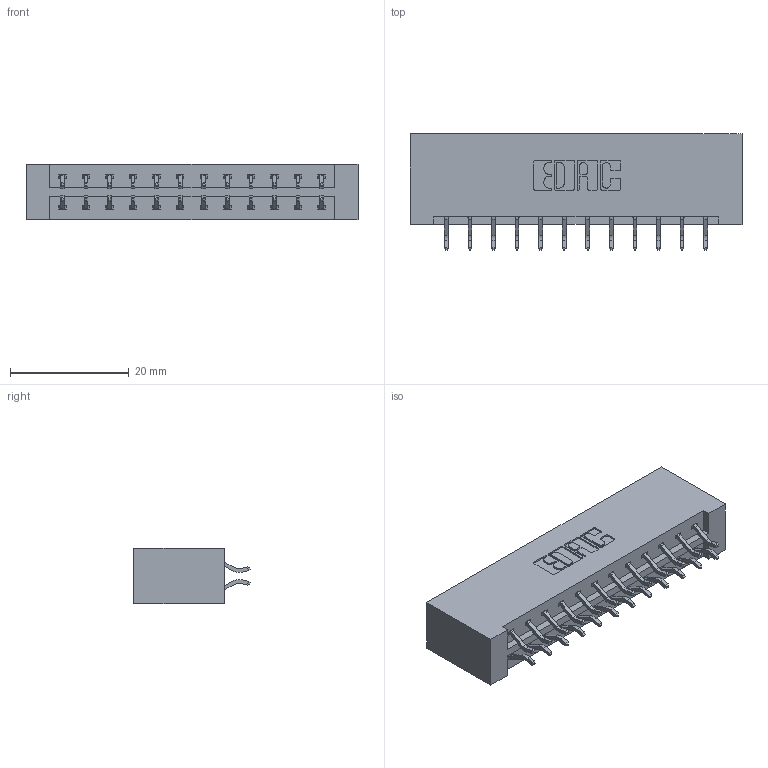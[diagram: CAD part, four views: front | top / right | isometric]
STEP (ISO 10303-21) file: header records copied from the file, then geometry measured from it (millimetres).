
FILE_DESCRIPTION (( 'STEP AP203' ), '1' );
FILE_NAME ('833-024-556-201.STEP', '2020-06-01T22:12:25', ( '' ), ( '' ), 'SwSTEP 2.0', 'SolidWorks 2020', '' );
FILE_SCHEMA (( 'CONFIG_CONTROL_DESIGN' ));
Length unit declared in the file: inch
Products named in the file (3): 833 Part_Lugless; 345-292-001_556 Tail; 833-024-556-201
Assembly tree (25 placements, depth 2):
  833-024-556-201
    833 Part_Lugless
    345-292-001_556 Tail  x24
Bounding box: 55.8 x 19.57 x 9.4 mm (x, y, z)
Volume: 6048 mm3; surface area: 6828.5 mm2
Topology: 25 solids, 25 shells, 1498 faces, 4439 edges, 2926 vertices
Faces by surface type: plane 1026, cylinder 472
Entity records: 11543 total; most frequent: CARTESIAN_POINT 1962, ORIENTED_EDGE 1886, DIRECTION 1711, EDGE_CURVE 943, LINE 815, VECTOR 815, VERTEX_POINT 626, AXIS2_PLACEMENT_3D 448
